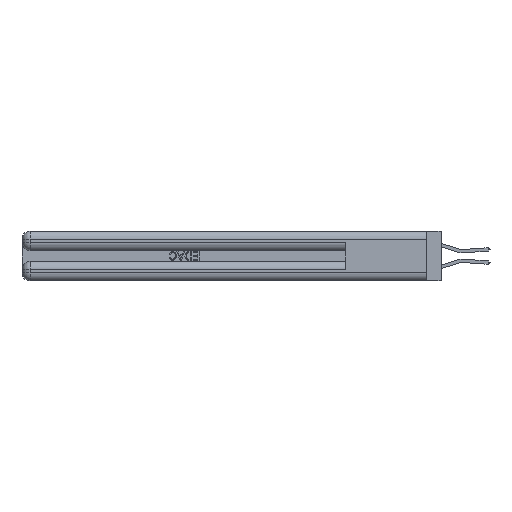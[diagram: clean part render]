
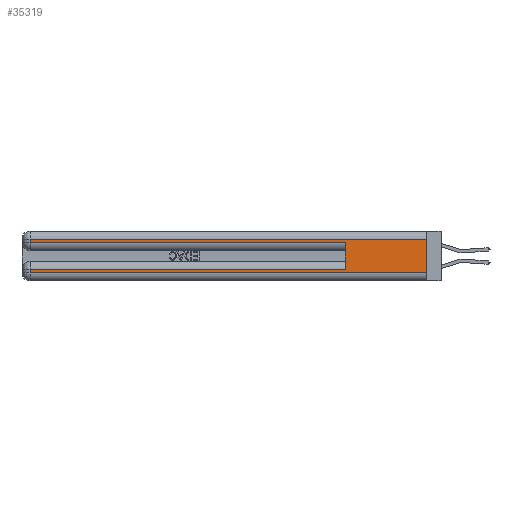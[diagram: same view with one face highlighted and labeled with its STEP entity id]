
A CAD part, left-side view. The second image highlights one B-rep face of the part: STEP entity #35319.
In plain terms, the highlighted planar face has unit normal (-1, 0, 0).
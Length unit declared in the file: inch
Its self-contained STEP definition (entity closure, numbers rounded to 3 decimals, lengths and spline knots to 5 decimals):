
#288 = EDGE_CURVE ( 'NONE', #7481, #16631, #11221, .T. ) ;
#782 = CARTESIAN_POINT ( 'NONE',  ( 0., 0., 0.285 ) ) ;
#989 = CARTESIAN_POINT ( 'NONE',  ( 0., 2.94, 0.085 ) ) ;
#1380 = ORIENTED_EDGE ( 'NONE', *, *, #15046, .T. ) ;
#1381 = VECTOR ( 'NONE', #24614, 39.37008 ) ;
#2122 = CARTESIAN_POINT ( 'NONE',  ( 0., 2.94, 0.37 ) ) ;
#4490 = LINE ( 'NONE', #2122, #1381 ) ;
#6502 = DIRECTION ( 'NONE',  ( 0., 0., 1. ) ) ;
#7034 = CARTESIAN_POINT ( 'NONE',  ( 0., 2.94, 0.285 ) ) ;
#7481 = VERTEX_POINT ( 'NONE', #9092 ) ;
#8253 = ORIENTED_EDGE ( 'NONE', *, *, #288, .T. ) ;
#8959 = CARTESIAN_POINT ( 'NONE',  ( 0., 0., 0.085 ) ) ;
#9066 = PLANE ( 'NONE',  #37122 ) ;
#9092 = CARTESIAN_POINT ( 'NONE',  ( 0., 2.94, 0.06 ) ) ;
#9965 = EDGE_CURVE ( 'NONE', #35206, #24304, #20855, .T. ) ;
#11221 = LINE ( 'NONE', #15251, #34703 ) ;
#13410 = EDGE_CURVE ( 'NONE', #24304, #31776, #42212, .T. ) ;
#13675 = CARTESIAN_POINT ( 'NONE',  ( 0., 0., 0.31 ) ) ;
#13948 = DIRECTION ( 'NONE',  ( 0., -1., 0. ) ) ;
#15046 = EDGE_CURVE ( 'NONE', #42037, #35206, #28846, .T. ) ;
#15053 = CARTESIAN_POINT ( 'NONE',  ( 0., 0., 0.06 ) ) ;
#15161 = VERTEX_POINT ( 'NONE', #20509 ) ;
#15251 = CARTESIAN_POINT ( 'NONE',  ( 0., 0., 0.06 ) ) ;
#15484 = DIRECTION ( 'NONE',  ( 0., 0., -1. ) ) ;
#16631 = VERTEX_POINT ( 'NONE', #15053 ) ;
#17156 = LINE ( 'NONE', #22270, #20689 ) ;
#18106 = VECTOR ( 'NONE', #23496, 39.37008 ) ;
#18371 = DIRECTION ( 'NONE',  ( 0., -1., 0. ) ) ;
#19667 = DIRECTION ( 'NONE',  ( 0., 0., -1. ) ) ;
#19864 = LINE ( 'NONE', #8959, #41357 ) ;
#20509 = CARTESIAN_POINT ( 'NONE',  ( 0., 0.6, 0.085 ) ) ;
#20689 = VECTOR ( 'NONE', #6502, 39.37008 ) ;
#20707 = EDGE_CURVE ( 'NONE', #40371, #7481, #4490, .T. ) ;
#20855 = LINE ( 'NONE', #39110, #34127 ) ;
#21713 = CARTESIAN_POINT ( 'NONE',  ( 0., 0., 0.37 ) ) ;
#22270 = CARTESIAN_POINT ( 'NONE',  ( 0., 0.6, 0.145 ) ) ;
#23496 = DIRECTION ( 'NONE',  ( 0., 1., 0. ) ) ;
#24304 = VERTEX_POINT ( 'NONE', #7034 ) ;
#24614 = DIRECTION ( 'NONE',  ( 0., 0., -1. ) ) ;
#27471 = ORIENTED_EDGE ( 'NONE', *, *, #9965, .T. ) ;
#28175 = DIRECTION ( 'NONE',  ( 1., 0., 0. ) ) ;
#28435 = DIRECTION ( 'NONE',  ( 0., 0., -1. ) ) ;
#28634 = DIRECTION ( 'NONE',  ( 0., 1., 0. ) ) ;
#28796 = ORIENTED_EDGE ( 'NONE', *, *, #13410, .T. ) ;
#28846 = LINE ( 'NONE', #13675, #18106 ) ;
#29115 = LINE ( 'NONE', #21713, #36723 ) ;
#29471 = VECTOR ( 'NONE', #13948, 39.37008 ) ;
#30143 = CARTESIAN_POINT ( 'NONE',  ( 0., 0.6, 0.285 ) ) ;
#31467 = EDGE_CURVE ( 'NONE', #15161, #40371, #19864, .T. ) ;
#31758 = CARTESIAN_POINT ( 'NONE',  ( 0., 0., 0.37 ) ) ;
#31776 = VERTEX_POINT ( 'NONE', #30143 ) ;
#34127 = VECTOR ( 'NONE', #19667, 39.37008 ) ;
#34148 = CARTESIAN_POINT ( 'NONE',  ( 0., 2.94, 0.31 ) ) ;
#34703 = VECTOR ( 'NONE', #18371, 39.37008 ) ;
#34874 = EDGE_LOOP ( 'NONE', ( #41960, #1380, #27471, #28796, #41757, #41087, #39593, #8253 ) ) ;
#35206 = VERTEX_POINT ( 'NONE', #34148 ) ;
#35319 = ADVANCED_FACE ( 'NONE', ( #38124 ), #9066, .F. ) ;
#36723 = VECTOR ( 'NONE', #28435, 39.37008 ) ;
#37122 = AXIS2_PLACEMENT_3D ( 'NONE', #31758, #28175, #15484 ) ;
#37947 = CARTESIAN_POINT ( 'NONE',  ( 0., 0., 0.31 ) ) ;
#38124 = FACE_OUTER_BOUND ( 'NONE', #34874, .T. ) ;
#38490 = EDGE_CURVE ( 'NONE', #15161, #31776, #17156, .T. ) ;
#39110 = CARTESIAN_POINT ( 'NONE',  ( 0., 2.94, 0.37 ) ) ;
#39593 = ORIENTED_EDGE ( 'NONE', *, *, #20707, .T. ) ;
#39983 = EDGE_CURVE ( 'NONE', #42037, #16631, #29115, .T. ) ;
#40371 = VERTEX_POINT ( 'NONE', #989 ) ;
#41087 = ORIENTED_EDGE ( 'NONE', *, *, #31467, .T. ) ;
#41357 = VECTOR ( 'NONE', #28634, 39.37008 ) ;
#41757 = ORIENTED_EDGE ( 'NONE', *, *, #38490, .F. ) ;
#41960 = ORIENTED_EDGE ( 'NONE', *, *, #39983, .F. ) ;
#42037 = VERTEX_POINT ( 'NONE', #37947 ) ;
#42212 = LINE ( 'NONE', #782, #29471 ) ;
